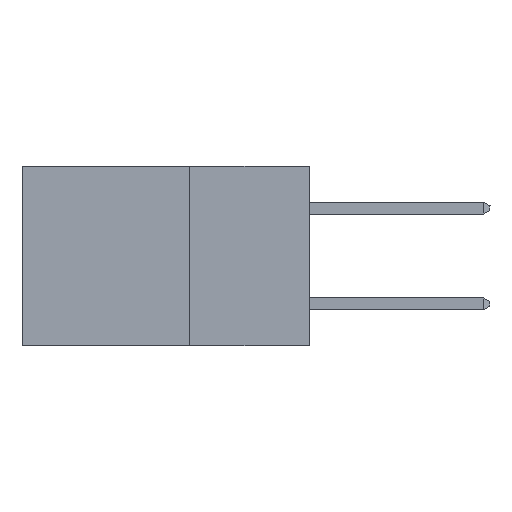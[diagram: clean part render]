
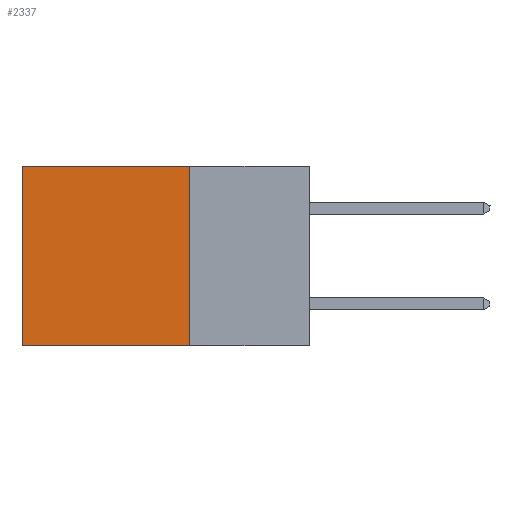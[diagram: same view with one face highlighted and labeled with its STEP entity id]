
A CAD part, left-side view. The second image highlights one B-rep face of the part: STEP entity #2337.
In plain terms, the highlighted planar face has unit normal (-1, 0, 0).
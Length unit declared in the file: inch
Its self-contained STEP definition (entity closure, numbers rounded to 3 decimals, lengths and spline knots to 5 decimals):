
#101 = EDGE_CURVE ( 'NONE', #804, #8526, #6856, .T. ) ;
#542 = CARTESIAN_POINT ( 'NONE',  ( 0.2875, 0.25, -0.375 ) ) ;
#587 = LINE ( 'NONE', #9889, #8364 ) ;
#658 = CARTESIAN_POINT ( 'NONE',  ( 0.2875, 0.6, 0. ) ) ;
#804 = VERTEX_POINT ( 'NONE', #11403 ) ;
#815 = ORIENTED_EDGE ( 'NONE', *, *, #2390, .F. ) ;
#2337 = ADVANCED_FACE ( 'NONE', ( #7014 ), #11186, .F. ) ;
#2390 = EDGE_CURVE ( 'NONE', #8526, #9232, #7988, .T. ) ;
#4312 = EDGE_CURVE ( 'NONE', #804, #4802, #11433, .T. ) ;
#4579 = DIRECTION ( 'NONE',  ( 1., 0., 0. ) ) ;
#4802 = VERTEX_POINT ( 'NONE', #658 ) ;
#4861 = CARTESIAN_POINT ( 'NONE',  ( 0.2875, 0.25, -0.375 ) ) ;
#6856 = LINE ( 'NONE', #542, #10533 ) ;
#6955 = EDGE_LOOP ( 'NONE', ( #8804, #815, #13633, #10252 ) ) ;
#7014 = FACE_OUTER_BOUND ( 'NONE', #6955, .T. ) ;
#7923 = DIRECTION ( 'NONE',  ( 0., 0., -1. ) ) ;
#7988 = LINE ( 'NONE', #4861, #10894 ) ;
#8225 = VECTOR ( 'NONE', #10257, 39.37008 ) ;
#8309 = CARTESIAN_POINT ( 'NONE',  ( 0.2875, 0.25, 0. ) ) ;
#8364 = VECTOR ( 'NONE', #8915, 39.37008 ) ;
#8526 = VERTEX_POINT ( 'NONE', #12929 ) ;
#8804 = ORIENTED_EDGE ( 'NONE', *, *, #11314, .T. ) ;
#8915 = DIRECTION ( 'NONE',  ( 0., 0., -1. ) ) ;
#9232 = VERTEX_POINT ( 'NONE', #12478 ) ;
#9840 = DIRECTION ( 'NONE',  ( 0., 0., -1. ) ) ;
#9889 = CARTESIAN_POINT ( 'NONE',  ( 0.2875, 0.6, -0.375 ) ) ;
#10003 = CARTESIAN_POINT ( 'NONE',  ( 0.2875, 0.25, -0.375 ) ) ;
#10252 = ORIENTED_EDGE ( 'NONE', *, *, #4312, .T. ) ;
#10257 = DIRECTION ( 'NONE',  ( 0., 1., 0. ) ) ;
#10533 = VECTOR ( 'NONE', #9840, 39.37008 ) ;
#10894 = VECTOR ( 'NONE', #11119, 39.37008 ) ;
#11119 = DIRECTION ( 'NONE',  ( 0., 1., 0. ) ) ;
#11186 = PLANE ( 'NONE',  #12876 ) ;
#11314 = EDGE_CURVE ( 'NONE', #4802, #9232, #587, .T. ) ;
#11403 = CARTESIAN_POINT ( 'NONE',  ( 0.2875, 0.25, 0. ) ) ;
#11433 = LINE ( 'NONE', #8309, #8225 ) ;
#12478 = CARTESIAN_POINT ( 'NONE',  ( 0.2875, 0.6, -0.375 ) ) ;
#12876 = AXIS2_PLACEMENT_3D ( 'NONE', #10003, #4579, #7923 ) ;
#12929 = CARTESIAN_POINT ( 'NONE',  ( 0.2875, 0.25, -0.375 ) ) ;
#13633 = ORIENTED_EDGE ( 'NONE', *, *, #101, .F. ) ;
